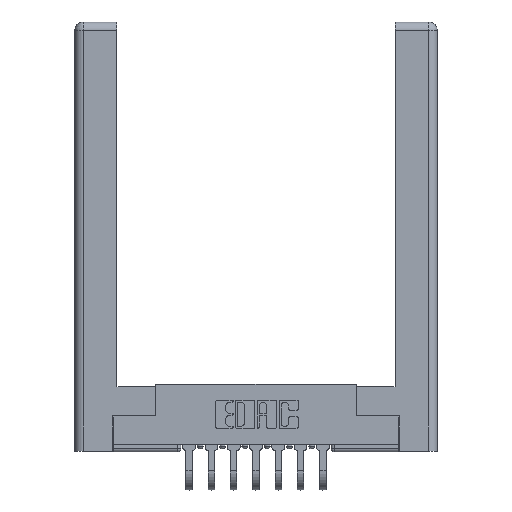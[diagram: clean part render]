
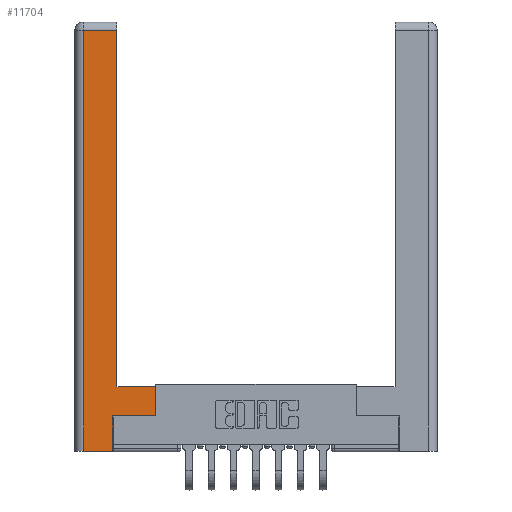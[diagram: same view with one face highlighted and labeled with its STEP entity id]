
A CAD part, top view. The second image highlights one B-rep face of the part: STEP entity #11704.
In plain terms, the highlighted planar face has unit normal (0, 0, 1).
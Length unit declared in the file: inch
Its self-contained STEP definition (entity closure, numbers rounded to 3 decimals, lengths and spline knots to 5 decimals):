
#79 = VECTOR ( 'NONE', #10351, 39.37008 ) ;
#100 = LINE ( 'NONE', #6334, #79 ) ;
#396 = LINE ( 'NONE', #4441, #7906 ) ;
#802 = EDGE_CURVE ( 'NONE', #9775, #3600, #10865, .T. ) ;
#883 = CARTESIAN_POINT ( 'NONE',  ( 0.265, 0.245, 0. ) ) ;
#992 = ORIENTED_EDGE ( 'NONE', *, *, #6690, .T. ) ;
#1078 = DIRECTION ( 'NONE',  ( 1., 0., 0. ) ) ;
#1450 = CARTESIAN_POINT ( 'NONE',  ( 0.295, 0.45, 0. ) ) ;
#1463 = ORIENTED_EDGE ( 'NONE', *, *, #6946, .T. ) ;
#1701 = CARTESIAN_POINT ( 'NONE',  ( 0.0615, 0., 0. ) ) ;
#1827 = DIRECTION ( 'NONE',  ( 0., -1., 0. ) ) ;
#1908 = LINE ( 'NONE', #13003, #2829 ) ;
#2020 = VERTEX_POINT ( 'NONE', #8606 ) ;
#2369 = EDGE_CURVE ( 'NONE', #2020, #4359, #1908, .T. ) ;
#2420 = VECTOR ( 'NONE', #10631, 39.37008 ) ;
#2594 = DIRECTION ( 'NONE',  ( 1., 0., 0. ) ) ;
#2775 = VERTEX_POINT ( 'NONE', #883 ) ;
#2829 = VECTOR ( 'NONE', #4881, 39.37008 ) ;
#3037 = EDGE_CURVE ( 'NONE', #2775, #4989, #8842, .T. ) ;
#3202 = EDGE_CURVE ( 'NONE', #4359, #4269, #7986, .T. ) ;
#3252 = VECTOR ( 'NONE', #1827, 39.37008 ) ;
#3266 = ORIENTED_EDGE ( 'NONE', *, *, #802, .T. ) ;
#3434 = EDGE_CURVE ( 'NONE', #4989, #2020, #396, .T. ) ;
#3472 = VERTEX_POINT ( 'NONE', #9602 ) ;
#3592 = CARTESIAN_POINT ( 'NONE',  ( 0.565, 0.245, 0. ) ) ;
#3600 = VERTEX_POINT ( 'NONE', #6822 ) ;
#3928 = VECTOR ( 'NONE', #2594, 39.37008 ) ;
#4269 = VERTEX_POINT ( 'NONE', #8331 ) ;
#4359 = VERTEX_POINT ( 'NONE', #1450 ) ;
#4441 = CARTESIAN_POINT ( 'NONE',  ( 0.565, 0.45, 0. ) ) ;
#4762 = CARTESIAN_POINT ( 'NONE',  ( 0.0615, 2.94, 0. ) ) ;
#4881 = DIRECTION ( 'NONE',  ( -1., 0., 0. ) ) ;
#4989 = VERTEX_POINT ( 'NONE', #10060 ) ;
#5775 = DIRECTION ( 'NONE',  ( -1., 0., 0. ) ) ;
#6107 = LINE ( 'NONE', #10131, #10828 ) ;
#6243 = CARTESIAN_POINT ( 'NONE',  ( 0.0615, 2.94, 0. ) ) ;
#6255 = FACE_OUTER_BOUND ( 'NONE', #11904, .T. ) ;
#6334 = CARTESIAN_POINT ( 'NONE',  ( 0.265, 0.245, 0. ) ) ;
#6625 = LINE ( 'NONE', #4762, #2420 ) ;
#6690 = EDGE_CURVE ( 'NONE', #3600, #3472, #6107, .T. ) ;
#6822 = CARTESIAN_POINT ( 'NONE',  ( 0.0615, 0., 0. ) ) ;
#6946 = EDGE_CURVE ( 'NONE', #4269, #9775, #6625, .T. ) ;
#7273 = ORIENTED_EDGE ( 'NONE', *, *, #3434, .T. ) ;
#7789 = PLANE ( 'NONE',  #9967 ) ;
#7906 = VECTOR ( 'NONE', #8495, 39.37008 ) ;
#7986 = LINE ( 'NONE', #11979, #11455 ) ;
#8308 = ORIENTED_EDGE ( 'NONE', *, *, #12981, .T. ) ;
#8331 = CARTESIAN_POINT ( 'NONE',  ( 0.295, 2.94, 0. ) ) ;
#8495 = DIRECTION ( 'NONE',  ( 0., 1., 0. ) ) ;
#8606 = CARTESIAN_POINT ( 'NONE',  ( 0.565, 0.45, 0. ) ) ;
#8702 = ORIENTED_EDGE ( 'NONE', *, *, #3202, .T. ) ;
#8842 = LINE ( 'NONE', #3592, #3928 ) ;
#9602 = CARTESIAN_POINT ( 'NONE',  ( 0.265, 0., 0. ) ) ;
#9775 = VERTEX_POINT ( 'NONE', #6243 ) ;
#9967 = AXIS2_PLACEMENT_3D ( 'NONE', #11645, #12642, #5775 ) ;
#10060 = CARTESIAN_POINT ( 'NONE',  ( 0.565, 0.245, 0. ) ) ;
#10131 = CARTESIAN_POINT ( 'NONE',  ( 0.265, 0., 0. ) ) ;
#10351 = DIRECTION ( 'NONE',  ( 0., 1., 0. ) ) ;
#10631 = DIRECTION ( 'NONE',  ( -1., 0., 0. ) ) ;
#10828 = VECTOR ( 'NONE', #1078, 39.37008 ) ;
#10865 = LINE ( 'NONE', #1701, #3252 ) ;
#11455 = VECTOR ( 'NONE', #12102, 39.37008 ) ;
#11645 = CARTESIAN_POINT ( 'NONE',  ( 0., 0., 0. ) ) ;
#11704 = ADVANCED_FACE ( 'NONE', ( #6255 ), #7789, .F. ) ;
#11718 = ORIENTED_EDGE ( 'NONE', *, *, #3037, .T. ) ;
#11904 = EDGE_LOOP ( 'NONE', ( #8702, #1463, #3266, #992, #8308, #11718, #7273, #12668 ) ) ;
#11979 = CARTESIAN_POINT ( 'NONE',  ( 0.295, 3., 0. ) ) ;
#12102 = DIRECTION ( 'NONE',  ( 0., 1., 0. ) ) ;
#12642 = DIRECTION ( 'NONE',  ( 0., 0., -1. ) ) ;
#12668 = ORIENTED_EDGE ( 'NONE', *, *, #2369, .T. ) ;
#12981 = EDGE_CURVE ( 'NONE', #3472, #2775, #100, .T. ) ;
#13003 = CARTESIAN_POINT ( 'NONE',  ( 0.295, 0.45, 0. ) ) ;
